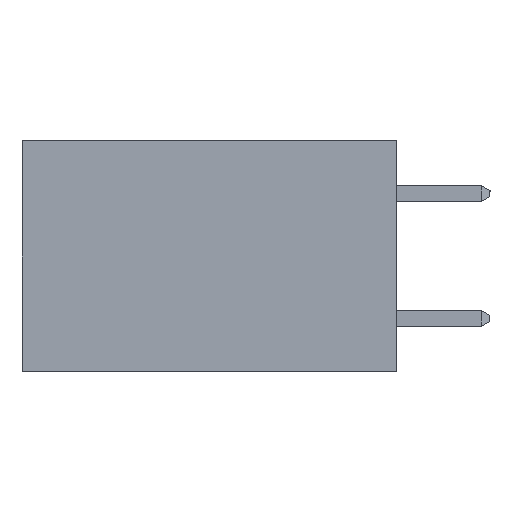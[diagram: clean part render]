
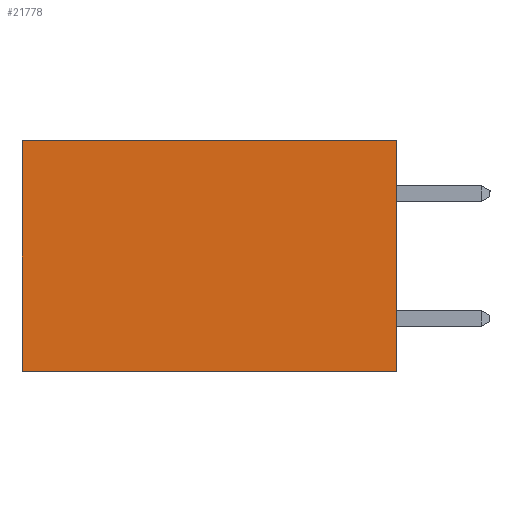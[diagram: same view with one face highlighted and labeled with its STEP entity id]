
A CAD part, left-side view. The second image highlights one B-rep face of the part: STEP entity #21778.
In plain terms, the highlighted planar face has unit normal (-1, 0, 0).
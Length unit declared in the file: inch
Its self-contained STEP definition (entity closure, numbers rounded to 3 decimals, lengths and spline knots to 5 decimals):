
#403 = VECTOR ( 'NONE', #4836, 39.37008 ) ;
#498 = VERTEX_POINT ( 'NONE', #16844 ) ;
#1174 = CARTESIAN_POINT ( 'NONE',  ( 0.2615, 0.6, 0. ) ) ;
#1981 = VERTEX_POINT ( 'NONE', #12728 ) ;
#2389 = EDGE_CURVE ( 'NONE', #18694, #16079, #8560, .T. ) ;
#4233 = AXIS2_PLACEMENT_3D ( 'NONE', #6216, #8280, #6105 ) ;
#4821 = DIRECTION ( 'NONE',  ( 0., 1., 0. ) ) ;
#4836 = DIRECTION ( 'NONE',  ( 0., 0., -1. ) ) ;
#5117 = PLANE ( 'NONE',  #4233 ) ;
#6065 = VECTOR ( 'NONE', #6605, 39.37008 ) ;
#6105 = DIRECTION ( 'NONE',  ( 0., 0., -1. ) ) ;
#6216 = CARTESIAN_POINT ( 'NONE',  ( 0.2615, 0., -0.37 ) ) ;
#6605 = DIRECTION ( 'NONE',  ( 0., 1., 0. ) ) ;
#8280 = DIRECTION ( 'NONE',  ( 1., 0., 0. ) ) ;
#8294 = VECTOR ( 'NONE', #9846, 39.37008 ) ;
#8560 = LINE ( 'NONE', #22323, #6065 ) ;
#8897 = ORIENTED_EDGE ( 'NONE', *, *, #14826, .T. ) ;
#9846 = DIRECTION ( 'NONE',  ( 0., 0., -1. ) ) ;
#10011 = LINE ( 'NONE', #10339, #16178 ) ;
#10061 = LINE ( 'NONE', #20493, #8294 ) ;
#10339 = CARTESIAN_POINT ( 'NONE',  ( 0.2615, 0., -0.37 ) ) ;
#10463 = CARTESIAN_POINT ( 'NONE',  ( 0.2615, 0.6, -0.37 ) ) ;
#11165 = ORIENTED_EDGE ( 'NONE', *, *, #2389, .T. ) ;
#12728 = CARTESIAN_POINT ( 'NONE',  ( 0.2615, 0.6, -0.37 ) ) ;
#14029 = EDGE_LOOP ( 'NONE', ( #8897, #20089, #20800, #11165 ) ) ;
#14826 = EDGE_CURVE ( 'NONE', #16079, #1981, #17220, .T. ) ;
#16079 = VERTEX_POINT ( 'NONE', #1174 ) ;
#16178 = VECTOR ( 'NONE', #4821, 39.37008 ) ;
#16774 = EDGE_CURVE ( 'NONE', #498, #1981, #10011, .T. ) ;
#16844 = CARTESIAN_POINT ( 'NONE',  ( 0.2615, 0., -0.37 ) ) ;
#17220 = LINE ( 'NONE', #10463, #403 ) ;
#18367 = FACE_OUTER_BOUND ( 'NONE', #14029, .T. ) ;
#18694 = VERTEX_POINT ( 'NONE', #21318 ) ;
#20089 = ORIENTED_EDGE ( 'NONE', *, *, #16774, .F. ) ;
#20493 = CARTESIAN_POINT ( 'NONE',  ( 0.2615, 0., -0.37 ) ) ;
#20800 = ORIENTED_EDGE ( 'NONE', *, *, #22204, .F. ) ;
#21318 = CARTESIAN_POINT ( 'NONE',  ( 0.2615, 0., 0. ) ) ;
#21778 = ADVANCED_FACE ( 'NONE', ( #18367 ), #5117, .F. ) ;
#22204 = EDGE_CURVE ( 'NONE', #18694, #498, #10061, .T. ) ;
#22323 = CARTESIAN_POINT ( 'NONE',  ( 0.2615, 0., 0. ) ) ;
